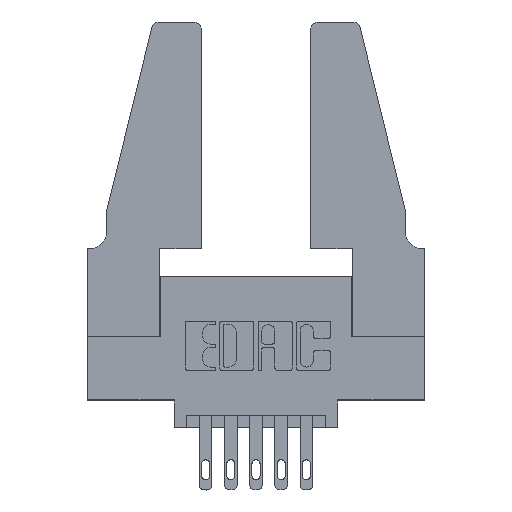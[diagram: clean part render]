
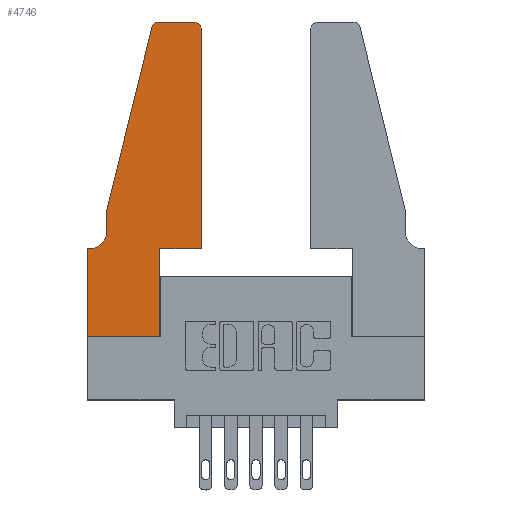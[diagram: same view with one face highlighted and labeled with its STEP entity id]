
A CAD part, top view. The second image highlights one B-rep face of the part: STEP entity #4746.
In plain terms, the highlighted planar face has unit normal (0, 0, 1).
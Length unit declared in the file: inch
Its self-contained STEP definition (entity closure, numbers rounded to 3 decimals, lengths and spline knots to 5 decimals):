
#38 = CARTESIAN_POINT ( 'NONE',  ( 0.0755, 0.5, 0.37 ) ) ;
#88 = CARTESIAN_POINT ( 'NONE',  ( 0.4505, 0.35, 0.37 ) ) ;
#95 = AXIS2_PLACEMENT_3D ( 'NONE', #5801, #3237, #739 ) ;
#97 = EDGE_CURVE ( 'NONE', #1028, #6568, #4226, .T. ) ;
#253 = ORIENTED_EDGE ( 'NONE', *, *, #97, .T. ) ;
#272 = LINE ( 'NONE', #446, #9379 ) ;
#405 = DIRECTION ( 'NONE',  ( -1., 0., 0. ) ) ;
#446 = CARTESIAN_POINT ( 'NONE',  ( 0.0755, 0.35, 0.37 ) ) ;
#739 = DIRECTION ( 'NONE',  ( 1., 0., 0. ) ) ;
#798 = CIRCLE ( 'NONE', #6908, 0.07 ) ;
#802 = ORIENTED_EDGE ( 'NONE', *, *, #7556, .T. ) ;
#819 = VERTEX_POINT ( 'NONE', #7270 ) ;
#1027 = VERTEX_POINT ( 'NONE', #3006 ) ;
#1028 = VERTEX_POINT ( 'NONE', #3954 ) ;
#1057 = CIRCLE ( 'NONE', #10886, 0.03 ) ;
#1162 = VECTOR ( 'NONE', #8775, 39.37008 ) ;
#1212 = DIRECTION ( 'NONE',  ( 1., 0., 0. ) ) ;
#1280 = ORIENTED_EDGE ( 'NONE', *, *, #10307, .T. ) ;
#1293 = VERTEX_POINT ( 'NONE', #9561 ) ;
#1361 = ORIENTED_EDGE ( 'NONE', *, *, #11099, .T. ) ;
#1463 = LINE ( 'NONE', #1903, #3329 ) ;
#1903 = CARTESIAN_POINT ( 'NONE',  ( 0.4505, 0.35, 0.37 ) ) ;
#2379 = CARTESIAN_POINT ( 'NONE',  ( 0.4205, 1.22, 0.37 ) ) ;
#2420 = EDGE_CURVE ( 'NONE', #4379, #6419, #8860, .T. ) ;
#2672 = ORIENTED_EDGE ( 'NONE', *, *, #9826, .T. ) ;
#2713 = CARTESIAN_POINT ( 'NONE',  ( 0.0755, 0.5, 0.37 ) ) ;
#2988 = VECTOR ( 'NONE', #9297, 39.37008 ) ;
#3006 = CARTESIAN_POINT ( 'NONE',  ( 0.0055, 0.35, 0.37 ) ) ;
#3018 = DIRECTION ( 'NONE',  ( 0., 0., -1. ) ) ;
#3153 = CARTESIAN_POINT ( 'NONE',  ( 0., 0.35, 0.37 ) ) ;
#3232 = DIRECTION ( 'NONE',  ( 0., 0., 1. ) ) ;
#3237 = DIRECTION ( 'NONE',  ( 0., 0., 1. ) ) ;
#3267 = CARTESIAN_POINT ( 'NONE',  ( 0.2605, 1.25, 0.37 ) ) ;
#3329 = VECTOR ( 'NONE', #3676, 39.37008 ) ;
#3603 = CARTESIAN_POINT ( 'NONE',  ( 0., 0., 0.37 ) ) ;
#3673 = EDGE_CURVE ( 'NONE', #1027, #9595, #272, .T. ) ;
#3676 = DIRECTION ( 'NONE',  ( 1., 0., 0. ) ) ;
#3790 = VERTEX_POINT ( 'NONE', #8357 ) ;
#3954 = CARTESIAN_POINT ( 'NONE',  ( 0.4205, 1.25, 0.37 ) ) ;
#4084 = CARTESIAN_POINT ( 'NONE',  ( 0.2865, 0.35, 0.37 ) ) ;
#4226 = LINE ( 'NONE', #3267, #2988 ) ;
#4227 = DIRECTION ( 'NONE',  ( 0., -1., 0. ) ) ;
#4273 = ORIENTED_EDGE ( 'NONE', *, *, #9715, .T. ) ;
#4359 = EDGE_LOOP ( 'NONE', ( #253, #1361, #802, #6778, #1280, #4894, #2672, #8668, #5841, #8727, #4273, #8903 ) ) ;
#4376 = CARTESIAN_POINT ( 'NONE',  ( 0., 0., 0.37 ) ) ;
#4379 = VERTEX_POINT ( 'NONE', #7108 ) ;
#4626 = VERTEX_POINT ( 'NONE', #4885 ) ;
#4699 = EDGE_CURVE ( 'NONE', #1293, #1028, #1057, .T. ) ;
#4746 = ADVANCED_FACE ( 'NONE', ( #9369 ), #5840, .T. ) ;
#4803 = DIRECTION ( 'NONE',  ( 0., 1., 0. ) ) ;
#4885 = CARTESIAN_POINT ( 'NONE',  ( 0.4505, 0.35, 0.37 ) ) ;
#4894 = ORIENTED_EDGE ( 'NONE', *, *, #3673, .T. ) ;
#5030 = VECTOR ( 'NONE', #4803, 39.37008 ) ;
#5179 = VECTOR ( 'NONE', #4227, 39.37008 ) ;
#5351 = VECTOR ( 'NONE', #9465, 39.37008 ) ;
#5482 = DIRECTION ( 'NONE',  ( 0., 1., 0. ) ) ;
#5537 = CIRCLE ( 'NONE', #10216, 0.03 ) ;
#5796 = CARTESIAN_POINT ( 'NONE',  ( 0.284, 1.22, 0.37 ) ) ;
#5801 = CARTESIAN_POINT ( 'NONE',  ( 0., 0.35, 0.37 ) ) ;
#5840 = PLANE ( 'NONE',  #95 ) ;
#5841 = ORIENTED_EDGE ( 'NONE', *, *, #11108, .T. ) ;
#6228 = LINE ( 'NONE', #88, #6637 ) ;
#6266 = CARTESIAN_POINT ( 'NONE',  ( 0.2865, 0., 0.37 ) ) ;
#6419 = VERTEX_POINT ( 'NONE', #6266 ) ;
#6496 = LINE ( 'NONE', #4376, #5179 ) ;
#6562 = DIRECTION ( 'NONE',  ( -1., 0., 0. ) ) ;
#6568 = VERTEX_POINT ( 'NONE', #11002 ) ;
#6637 = VECTOR ( 'NONE', #5482, 39.37008 ) ;
#6778 = ORIENTED_EDGE ( 'NONE', *, *, #10715, .T. ) ;
#6908 = AXIS2_PLACEMENT_3D ( 'NONE', #9197, #3018, #6562 ) ;
#6920 = DIRECTION ( 'NONE',  ( 0., 0., 1. ) ) ;
#7084 = VERTEX_POINT ( 'NONE', #38 ) ;
#7108 = CARTESIAN_POINT ( 'NONE',  ( 0., 0., 0.37 ) ) ;
#7270 = CARTESIAN_POINT ( 'NONE',  ( 0.2865, 0.35, 0.37 ) ) ;
#7556 = EDGE_CURVE ( 'NONE', #10983, #7084, #9415, .T. ) ;
#8357 = CARTESIAN_POINT ( 'NONE',  ( 0.0755, 0.42, 0.37 ) ) ;
#8526 = EDGE_CURVE ( 'NONE', #819, #4626, #1463, .T. ) ;
#8668 = ORIENTED_EDGE ( 'NONE', *, *, #2420, .T. ) ;
#8716 = DIRECTION ( 'NONE',  ( 1., 0., 0. ) ) ;
#8727 = ORIENTED_EDGE ( 'NONE', *, *, #8526, .T. ) ;
#8775 = DIRECTION ( 'NONE',  ( 0., -1., 0. ) ) ;
#8845 = CARTESIAN_POINT ( 'NONE',  ( 0.0755, 0.5, 0.37 ) ) ;
#8860 = LINE ( 'NONE', #3603, #10780 ) ;
#8903 = ORIENTED_EDGE ( 'NONE', *, *, #4699, .T. ) ;
#9066 = LINE ( 'NONE', #4084, #5030 ) ;
#9197 = CARTESIAN_POINT ( 'NONE',  ( 0.0055, 0.42, 0.37 ) ) ;
#9266 = DIRECTION ( 'NONE',  ( 1., 0., 0. ) ) ;
#9297 = DIRECTION ( 'NONE',  ( -1., 0., 0. ) ) ;
#9369 = FACE_OUTER_BOUND ( 'NONE', #4359, .T. ) ;
#9379 = VECTOR ( 'NONE', #405, 39.37008 ) ;
#9415 = LINE ( 'NONE', #2713, #5351 ) ;
#9465 = DIRECTION ( 'NONE',  ( -0.239, -0.971, 0. ) ) ;
#9561 = CARTESIAN_POINT ( 'NONE',  ( 0.4505, 1.22, 0.37 ) ) ;
#9595 = VERTEX_POINT ( 'NONE', #3153 ) ;
#9715 = EDGE_CURVE ( 'NONE', #4626, #1293, #6228, .T. ) ;
#9796 = CARTESIAN_POINT ( 'NONE',  ( 0.25487, 1.22718, 0.37 ) ) ;
#9826 = EDGE_CURVE ( 'NONE', #9595, #4379, #6496, .T. ) ;
#10042 = LINE ( 'NONE', #8845, #1162 ) ;
#10216 = AXIS2_PLACEMENT_3D ( 'NONE', #5796, #3232, #9266 ) ;
#10307 = EDGE_CURVE ( 'NONE', #3790, #1027, #798, .T. ) ;
#10715 = EDGE_CURVE ( 'NONE', #7084, #3790, #10042, .T. ) ;
#10780 = VECTOR ( 'NONE', #8716, 39.37008 ) ;
#10886 = AXIS2_PLACEMENT_3D ( 'NONE', #2379, #6920, #1212 ) ;
#10983 = VERTEX_POINT ( 'NONE', #9796 ) ;
#11002 = CARTESIAN_POINT ( 'NONE',  ( 0.284, 1.25, 0.37 ) ) ;
#11099 = EDGE_CURVE ( 'NONE', #6568, #10983, #5537, .T. ) ;
#11108 = EDGE_CURVE ( 'NONE', #6419, #819, #9066, .T. ) ;
